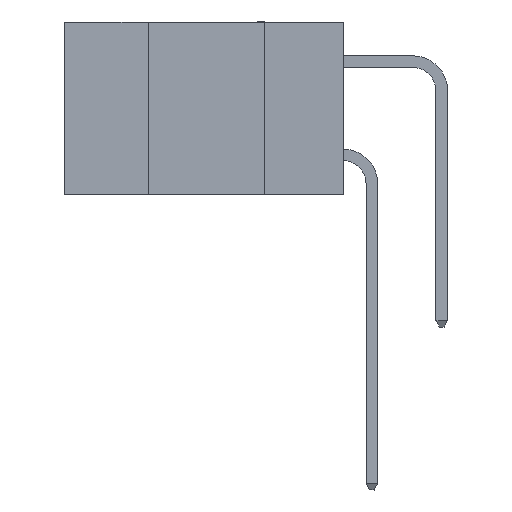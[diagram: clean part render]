
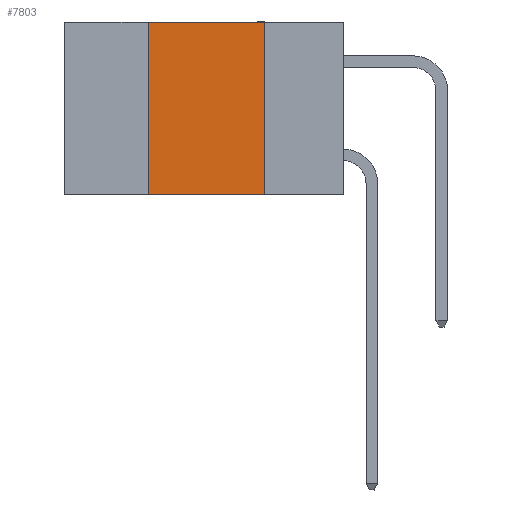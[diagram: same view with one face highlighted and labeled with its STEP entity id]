
A CAD part, left-side view. The second image highlights one B-rep face of the part: STEP entity #7803.
In plain terms, the highlighted planar face has unit normal (-1, 0, 0).
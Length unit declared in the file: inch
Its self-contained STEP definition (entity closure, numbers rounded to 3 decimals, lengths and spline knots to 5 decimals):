
#915 = DIRECTION ( 'NONE',  ( 0., -1., 0. ) ) ;
#1244 = AXIS2_PLACEMENT_3D ( 'NONE', #15235, #1886, #17512 ) ;
#1886 = DIRECTION ( 'NONE',  ( 1., 0., 0. ) ) ;
#2725 = CARTESIAN_POINT ( 'NONE',  ( 0., 0.6, -0.37 ) ) ;
#3942 = ORIENTED_EDGE ( 'NONE', *, *, #23157, .T. ) ;
#4840 = EDGE_CURVE ( 'NONE', #12744, #9337, #14347, .T. ) ;
#4955 = DIRECTION ( 'NONE',  ( 0., -1., 0. ) ) ;
#5243 = EDGE_CURVE ( 'NONE', #25655, #24290, #10506, .T. ) ;
#7085 = DIRECTION ( 'NONE',  ( 0., 0., 1. ) ) ;
#7617 = CARTESIAN_POINT ( 'NONE',  ( 0., 0.6, 0. ) ) ;
#7803 = ADVANCED_FACE ( 'NONE', ( #22899 ), #24071, .F. ) ;
#9337 = VERTEX_POINT ( 'NONE', #22953 ) ;
#9551 = CARTESIAN_POINT ( 'NONE',  ( 0., 0.17, 0. ) ) ;
#10506 = LINE ( 'NONE', #24497, #14317 ) ;
#11413 = LINE ( 'NONE', #2725, #22600 ) ;
#11943 = LINE ( 'NONE', #7617, #16500 ) ;
#12744 = VERTEX_POINT ( 'NONE', #23211 ) ;
#14317 = VECTOR ( 'NONE', #7085, 39.37008 ) ;
#14347 = LINE ( 'NONE', #9551, #18921 ) ;
#15235 = CARTESIAN_POINT ( 'NONE',  ( 0., 0.6, 0. ) ) ;
#15563 = EDGE_LOOP ( 'NONE', ( #23674, #20705, #26411, #3942 ) ) ;
#15598 = DIRECTION ( 'NONE',  ( 0., 0., -1. ) ) ;
#16500 = VECTOR ( 'NONE', #915, 39.37008 ) ;
#17512 = DIRECTION ( 'NONE',  ( 0., 0., -1. ) ) ;
#18921 = VECTOR ( 'NONE', #15598, 39.37008 ) ;
#20705 = ORIENTED_EDGE ( 'NONE', *, *, #26375, .F. ) ;
#21917 = CARTESIAN_POINT ( 'NONE',  ( 0., 0.42, -0.37 ) ) ;
#22600 = VECTOR ( 'NONE', #4955, 39.37008 ) ;
#22899 = FACE_OUTER_BOUND ( 'NONE', #15563, .T. ) ;
#22953 = CARTESIAN_POINT ( 'NONE',  ( 0., 0.17, -0.37 ) ) ;
#23157 = EDGE_CURVE ( 'NONE', #25655, #9337, #11413, .T. ) ;
#23211 = CARTESIAN_POINT ( 'NONE',  ( 0., 0.17, 0. ) ) ;
#23674 = ORIENTED_EDGE ( 'NONE', *, *, #4840, .F. ) ;
#24071 = PLANE ( 'NONE',  #1244 ) ;
#24290 = VERTEX_POINT ( 'NONE', #28532 ) ;
#24497 = CARTESIAN_POINT ( 'NONE',  ( 0., 0.42, 0. ) ) ;
#25655 = VERTEX_POINT ( 'NONE', #21917 ) ;
#26375 = EDGE_CURVE ( 'NONE', #24290, #12744, #11943, .T. ) ;
#26411 = ORIENTED_EDGE ( 'NONE', *, *, #5243, .F. ) ;
#28532 = CARTESIAN_POINT ( 'NONE',  ( 0., 0.42, 0. ) ) ;
